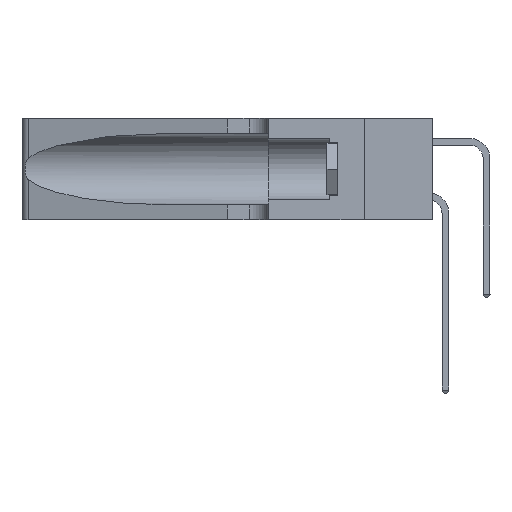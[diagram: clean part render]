
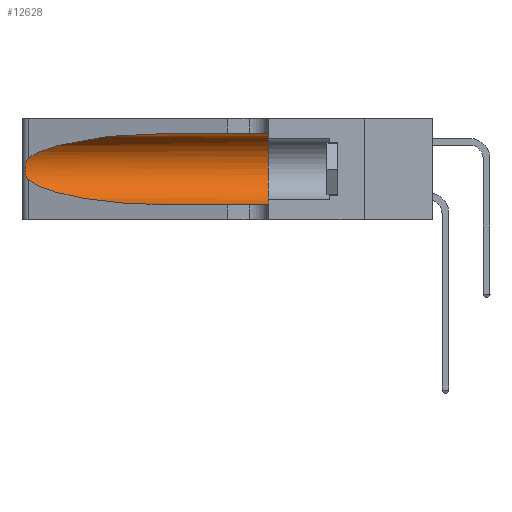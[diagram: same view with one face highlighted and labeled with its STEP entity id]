
A CAD part, left-side view. The second image highlights one B-rep face of the part: STEP entity #12628.
In plain terms, the highlighted cylindrical face has radius 3.308 mm (diameter 6.617 mm), a partial arc.
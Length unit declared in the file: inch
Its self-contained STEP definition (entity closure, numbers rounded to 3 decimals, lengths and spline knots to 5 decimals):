
#177 = ORIENTED_EDGE ( 'NONE', *, *, #11296, .T. ) ;
#1209 = EDGE_LOOP ( 'NONE', ( #17376, #13726, #177, #19545, #13163, #3084 ) ) ;
#1340 = VERTEX_POINT ( 'NONE', #21654 ) ;
#1737 = B_SPLINE_CURVE_WITH_KNOTS ( 'NONE', 3,
 ( #13122, #5506, #20644, #9356, #22484, #11270, #24349, #13202, #1818, #15104, #3698, #16956, #5583, #18826 ),
 .UNSPECIFIED., .F., .F.,
 ( 4, 2, 2, 2, 2, 2, 4 ),
 ( 0., 0.00027, 0.00053, 0.00107, 0.0016, 0.00187, 0.00214 ),
 .UNSPECIFIED. ) ;
#1818 = CARTESIAN_POINT ( 'NONE',  ( 0.26017, 1.23833, 0.17102 ) ) ;
#1879 =( BOUNDED_CURVE ( )  B_SPLINE_CURVE ( 3, ( #19536, #2512, #2598, #15874 ),
 .UNSPECIFIED., .F., .T. ) 
 B_SPLINE_CURVE_WITH_KNOTS ( ( 4, 4 ),
 ( 3.44316, 4.71239 ),
 .UNSPECIFIED. ) 
 CURVE ( )  GEOMETRIC_REPRESENTATION_ITEM ( )  RATIONAL_B_SPLINE_CURVE ( ( 1., 0.87, 0.87, 1. ) ) 
 REPRESENTATION_ITEM ( '' )  );
#2140 = CARTESIAN_POINT ( 'NONE',  ( 0.1305, 0.35, 0.185 ) ) ;
#2512 = CARTESIAN_POINT ( 'NONE',  ( 0.2373, 1.15595, 0.08982 ) ) ;
#2598 = CARTESIAN_POINT ( 'NONE',  ( 0.18966, 0.96281, 0.05475 ) ) ;
#2814 = VERTEX_POINT ( 'NONE', #10769 ) ;
#3084 = ORIENTED_EDGE ( 'NONE', *, *, #9924, .F. ) ;
#3383 =( BOUNDED_CURVE ( )  B_SPLINE_CURVE ( 3, ( #16943, #20709, #9426, #22551 ),
 .UNSPECIFIED., .F., .F. ) 
 B_SPLINE_CURVE_WITH_KNOTS ( ( 4, 4 ),
 ( 1.5708, 2.84003 ),
 .UNSPECIFIED. ) 
 CURVE ( )  GEOMETRIC_REPRESENTATION_ITEM ( )  RATIONAL_B_SPLINE_CURVE ( ( 1., 0.87, 0.87, 1. ) ) 
 REPRESENTATION_ITEM ( '' )  );
#3698 = CARTESIAN_POINT ( 'NONE',  ( 0.25789, 1.23486, 0.15765 ) ) ;
#4007 = DIRECTION ( 'NONE',  ( 0., 0., 1. ) ) ;
#4107 = DIRECTION ( 'NONE',  ( 0., -1., 0. ) ) ;
#4532 = EDGE_CURVE ( 'NONE', #1340, #9789, #3383, .T. ) ;
#4742 = DIRECTION ( 'NONE',  ( 0., 0., -1. ) ) ;
#4774 = VERTEX_POINT ( 'NONE', #21336 ) ;
#5506 = CARTESIAN_POINT ( 'NONE',  ( 0.25555, 1.22994, 0.2215 ) ) ;
#5527 = EDGE_CURVE ( 'NONE', #21049, #4774, #15067, .T. ) ;
#5583 = CARTESIAN_POINT ( 'NONE',  ( 0.25555, 1.22993, 0.14849 ) ) ;
#5869 = CYLINDRICAL_SURFACE ( 'NONE', #8149, 0.13025 ) ;
#6566 = CARTESIAN_POINT ( 'NONE',  ( 0.1305, 1.61858, 0.185 ) ) ;
#8149 = AXIS2_PLACEMENT_3D ( 'NONE', #6566, #16155, #4742 ) ;
#9274 = CIRCLE ( 'NONE', #21232, 0.13025 ) ;
#9356 = CARTESIAN_POINT ( 'NONE',  ( 0.25787, 1.23484, 0.2124 ) ) ;
#9426 = CARTESIAN_POINT ( 'NONE',  ( 0.2373, 1.15595, 0.28018 ) ) ;
#9789 = VERTEX_POINT ( 'NONE', #18838 ) ;
#9924 = EDGE_CURVE ( 'NONE', #1340, #20624, #19934, .T. ) ;
#9996 = VECTOR ( 'NONE', #12140, 39.37008 ) ;
#10475 = EDGE_CURVE ( 'NONE', #20624, #4774, #9274, .T. ) ;
#10769 = CARTESIAN_POINT ( 'NONE',  ( 0.25487, 1.22718, 0.14631 ) ) ;
#11270 = CARTESIAN_POINT ( 'NONE',  ( 0.26018, 1.23835, 0.19895 ) ) ;
#11296 = EDGE_CURVE ( 'NONE', #2814, #21049, #1879, .T. ) ;
#12140 = DIRECTION ( 'NONE',  ( 0., -1., 0. ) ) ;
#12231 = EDGE_CURVE ( 'NONE', #9789, #2814, #1737, .T. ) ;
#12628 = ADVANCED_FACE ( 'NONE', ( #20959 ), #5869, .F. ) ;
#13122 = CARTESIAN_POINT ( 'NONE',  ( 0.25487, 1.22718, 0.22369 ) ) ;
#13163 = ORIENTED_EDGE ( 'NONE', *, *, #10475, .F. ) ;
#13202 = CARTESIAN_POINT ( 'NONE',  ( 0.26075, 1.23896, 0.178 ) ) ;
#13726 = ORIENTED_EDGE ( 'NONE', *, *, #12231, .T. ) ;
#14966 = VECTOR ( 'NONE', #4107, 39.37008 ) ;
#15067 = LINE ( 'NONE', #21468, #9996 ) ;
#15104 = CARTESIAN_POINT ( 'NONE',  ( 0.25856, 1.23593, 0.16098 ) ) ;
#15427 = DIRECTION ( 'NONE',  ( 0., 1., 0. ) ) ;
#15874 = CARTESIAN_POINT ( 'NONE',  ( 0.1305, 0.72297, 0.05475 ) ) ;
#16155 = DIRECTION ( 'NONE',  ( 0., -1., 0. ) ) ;
#16943 = CARTESIAN_POINT ( 'NONE',  ( 0.1305, 0.72297, 0.31525 ) ) ;
#16956 = CARTESIAN_POINT ( 'NONE',  ( 0.25639, 1.23186, 0.15144 ) ) ;
#17376 = ORIENTED_EDGE ( 'NONE', *, *, #4532, .T. ) ;
#18826 = CARTESIAN_POINT ( 'NONE',  ( 0.25487, 1.22718, 0.14631 ) ) ;
#18838 = CARTESIAN_POINT ( 'NONE',  ( 0.25487, 1.22718, 0.22369 ) ) ;
#19536 = CARTESIAN_POINT ( 'NONE',  ( 0.25487, 1.22718, 0.14631 ) ) ;
#19545 = ORIENTED_EDGE ( 'NONE', *, *, #5527, .T. ) ;
#19837 = CARTESIAN_POINT ( 'NONE',  ( 0.1305, 0.72297, 0.05475 ) ) ;
#19934 = LINE ( 'NONE', #22888, #14966 ) ;
#20624 = VERTEX_POINT ( 'NONE', #24210 ) ;
#20644 = CARTESIAN_POINT ( 'NONE',  ( 0.25639, 1.23184, 0.21858 ) ) ;
#20709 = CARTESIAN_POINT ( 'NONE',  ( 0.18966, 0.96281, 0.31525 ) ) ;
#20959 = FACE_OUTER_BOUND ( 'NONE', #1209, .T. ) ;
#21049 = VERTEX_POINT ( 'NONE', #19837 ) ;
#21232 = AXIS2_PLACEMENT_3D ( 'NONE', #2140, #15427, #4007 ) ;
#21336 = CARTESIAN_POINT ( 'NONE',  ( 0.1305, 0.35, 0.05475 ) ) ;
#21468 = CARTESIAN_POINT ( 'NONE',  ( 0.1305, 1.61858, 0.05475 ) ) ;
#21654 = CARTESIAN_POINT ( 'NONE',  ( 0.1305, 0.72297, 0.31525 ) ) ;
#22484 = CARTESIAN_POINT ( 'NONE',  ( 0.25854, 1.2359, 0.20912 ) ) ;
#22551 = CARTESIAN_POINT ( 'NONE',  ( 0.25487, 1.22718, 0.22369 ) ) ;
#22888 = CARTESIAN_POINT ( 'NONE',  ( 0.1305, 1.61858, 0.31525 ) ) ;
#24210 = CARTESIAN_POINT ( 'NONE',  ( 0.1305, 0.35, 0.31525 ) ) ;
#24349 = CARTESIAN_POINT ( 'NONE',  ( 0.26075, 1.23896, 0.19203 ) ) ;
